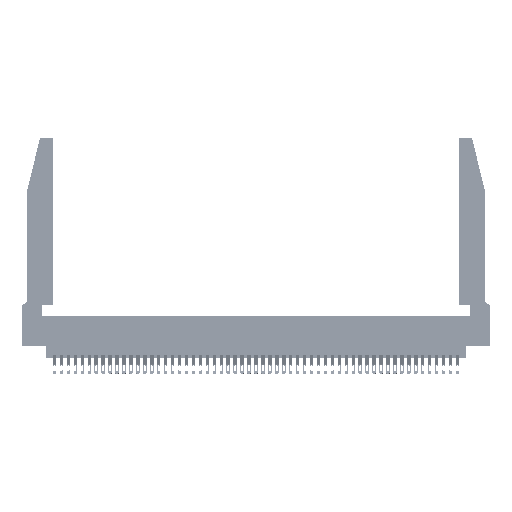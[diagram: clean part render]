
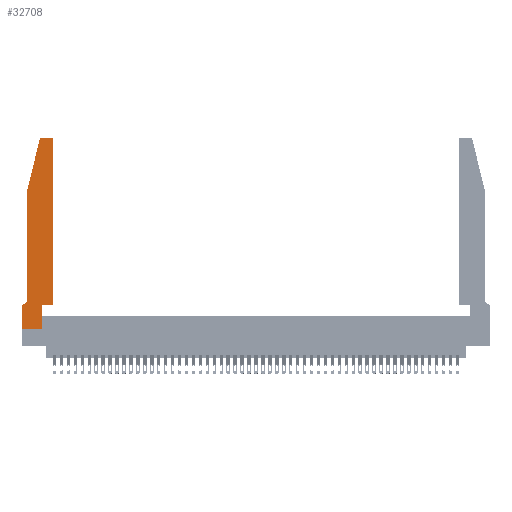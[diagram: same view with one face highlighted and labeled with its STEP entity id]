
A CAD part, top view. The second image highlights one B-rep face of the part: STEP entity #32708.
In plain terms, the highlighted planar face has unit normal (0, 0, 1).
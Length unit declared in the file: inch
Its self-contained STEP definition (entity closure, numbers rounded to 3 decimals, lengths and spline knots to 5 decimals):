
#137 = VERTEX_POINT ( 'NONE', #3479 ) ;
#506 = ORIENTED_EDGE ( 'NONE', *, *, #31045, .T. ) ;
#1207 = DIRECTION ( 'NONE',  ( 1., 0., 0. ) ) ;
#2155 = CARTESIAN_POINT ( 'NONE',  ( 0.0755, 2., 0.37 ) ) ;
#3479 = CARTESIAN_POINT ( 'NONE',  ( 0.2865, 0., 0.37 ) ) ;
#3508 = EDGE_CURVE ( 'NONE', #137, #24371, #4201, .T. ) ;
#4201 = LINE ( 'NONE', #27935, #20249 ) ;
#4368 = CARTESIAN_POINT ( 'NONE',  ( 0.0755, 2., 0.37 ) ) ;
#4693 = CARTESIAN_POINT ( 'NONE',  ( 0.0755, 0.42, 0.37 ) ) ;
#5701 = CARTESIAN_POINT ( 'NONE',  ( 0.0755, 2., 0.37 ) ) ;
#6188 = AXIS2_PLACEMENT_3D ( 'NONE', #13835, #40429, #44256 ) ;
#6487 = AXIS2_PLACEMENT_3D ( 'NONE', #41395, #21757, #26065 ) ;
#7069 = LINE ( 'NONE', #2155, #46385 ) ;
#8579 = CARTESIAN_POINT ( 'NONE',  ( 0.2865, 0.35, 0.37 ) ) ;
#10201 = CIRCLE ( 'NONE', #35204, 0.03 ) ;
#10376 = VECTOR ( 'NONE', #1207, 39.37008 ) ;
#10714 = CIRCLE ( 'NONE', #6188, 0.03 ) ;
#11457 = VERTEX_POINT ( 'NONE', #45460 ) ;
#11647 = LINE ( 'NONE', #43375, #15791 ) ;
#12059 = FACE_OUTER_BOUND ( 'NONE', #23910, .T. ) ;
#12420 = ORIENTED_EDGE ( 'NONE', *, *, #34769, .T. ) ;
#13361 = DIRECTION ( 'NONE',  ( 0., -1., 0. ) ) ;
#13835 = CARTESIAN_POINT ( 'NONE',  ( 0.4205, 2.72, 0.37 ) ) ;
#13990 = EDGE_CURVE ( 'NONE', #24371, #29983, #34779, .T. ) ;
#15791 = VECTOR ( 'NONE', #46891, 39.37008 ) ;
#15926 = VERTEX_POINT ( 'NONE', #24066 ) ;
#16414 = ORIENTED_EDGE ( 'NONE', *, *, #20562, .T. ) ;
#17161 = CARTESIAN_POINT ( 'NONE',  ( 0.4205, 2.75, 0.37 ) ) ;
#17663 = ORIENTED_EDGE ( 'NONE', *, *, #47077, .T. ) ;
#17779 = VERTEX_POINT ( 'NONE', #45844 ) ;
#18702 = CARTESIAN_POINT ( 'NONE',  ( 0.4505, 0.35, 0.37 ) ) ;
#19654 = VERTEX_POINT ( 'NONE', #4368 ) ;
#19939 = CARTESIAN_POINT ( 'NONE',  ( 0., 0., 0.37 ) ) ;
#20249 = VECTOR ( 'NONE', #40398, 39.37008 ) ;
#20545 = CARTESIAN_POINT ( 'NONE',  ( 0., 0., 0.37 ) ) ;
#20562 = EDGE_CURVE ( 'NONE', #17779, #137, #39783, .T. ) ;
#21757 = DIRECTION ( 'NONE',  ( 0., 0., -1. ) ) ;
#21945 = EDGE_CURVE ( 'NONE', #29983, #27282, #43775, .T. ) ;
#22101 = DIRECTION ( 'NONE',  ( 0., 0., 1. ) ) ;
#22217 = EDGE_CURVE ( 'NONE', #28894, #11457, #11647, .T. ) ;
#22573 = DIRECTION ( 'NONE',  ( 0., 1., 0. ) ) ;
#23110 = VECTOR ( 'NONE', #39688, 39.37008 ) ;
#23624 = CIRCLE ( 'NONE', #6487, 0.07 ) ;
#23910 = EDGE_LOOP ( 'NONE', ( #25880, #29594, #12420, #30678, #506, #31375, #17663, #16414, #26755, #45227, #28494, #25932 ) ) ;
#24066 = CARTESIAN_POINT ( 'NONE',  ( 0., 0.35, 0.37 ) ) ;
#24371 = VERTEX_POINT ( 'NONE', #8579 ) ;
#25573 = PLANE ( 'NONE',  #31054 ) ;
#25880 = ORIENTED_EDGE ( 'NONE', *, *, #22217, .T. ) ;
#25932 = ORIENTED_EDGE ( 'NONE', *, *, #29044, .T. ) ;
#26065 = DIRECTION ( 'NONE',  ( -1., 0., 0. ) ) ;
#26755 = ORIENTED_EDGE ( 'NONE', *, *, #3508, .T. ) ;
#27097 = VERTEX_POINT ( 'NONE', #4693 ) ;
#27282 = VERTEX_POINT ( 'NONE', #33248 ) ;
#27413 = CARTESIAN_POINT ( 'NONE',  ( 0.4505, 0.35, 0.37 ) ) ;
#27922 = LINE ( 'NONE', #5701, #40997 ) ;
#27935 = CARTESIAN_POINT ( 'NONE',  ( 0.2865, 0.35, 0.37 ) ) ;
#28453 = EDGE_CURVE ( 'NONE', #11457, #29487, #10201, .T. ) ;
#28494 = ORIENTED_EDGE ( 'NONE', *, *, #21945, .T. ) ;
#28683 = DIRECTION ( 'NONE',  ( -0.239, -0.971, 0. ) ) ;
#28894 = VERTEX_POINT ( 'NONE', #17161 ) ;
#28906 = CARTESIAN_POINT ( 'NONE',  ( 0.284, 2.72, 0.37 ) ) ;
#29044 = EDGE_CURVE ( 'NONE', #27282, #28894, #10714, .T. ) ;
#29487 = VERTEX_POINT ( 'NONE', #38893 ) ;
#29594 = ORIENTED_EDGE ( 'NONE', *, *, #28453, .T. ) ;
#29671 = VERTEX_POINT ( 'NONE', #39714 ) ;
#29983 = VERTEX_POINT ( 'NONE', #18702 ) ;
#30678 = ORIENTED_EDGE ( 'NONE', *, *, #34431, .T. ) ;
#31045 = EDGE_CURVE ( 'NONE', #27097, #29671, #23624, .T. ) ;
#31054 = AXIS2_PLACEMENT_3D ( 'NONE', #33600, #22101, #44415 ) ;
#31074 = VECTOR ( 'NONE', #42930, 39.37008 ) ;
#31375 = ORIENTED_EDGE ( 'NONE', *, *, #38452, .T. ) ;
#32708 = ADVANCED_FACE ( 'NONE', ( #12059 ), #25573, .T. ) ;
#33248 = CARTESIAN_POINT ( 'NONE',  ( 0.4505, 2.72, 0.37 ) ) ;
#33600 = CARTESIAN_POINT ( 'NONE',  ( 0., 0.35, 0.37 ) ) ;
#34431 = EDGE_CURVE ( 'NONE', #19654, #27097, #27922, .T. ) ;
#34582 = CARTESIAN_POINT ( 'NONE',  ( 0.0755, 0.35, 0.37 ) ) ;
#34769 = EDGE_CURVE ( 'NONE', #29487, #19654, #7069, .T. ) ;
#34779 = LINE ( 'NONE', #27413, #10376 ) ;
#35204 = AXIS2_PLACEMENT_3D ( 'NONE', #28906, #44389, #47580 ) ;
#37215 = VECTOR ( 'NONE', #22573, 39.37008 ) ;
#38452 = EDGE_CURVE ( 'NONE', #29671, #15926, #47821, .T. ) ;
#38893 = CARTESIAN_POINT ( 'NONE',  ( 0.25487, 2.72718, 0.37 ) ) ;
#39688 = DIRECTION ( 'NONE',  ( 1., 0., 0. ) ) ;
#39714 = CARTESIAN_POINT ( 'NONE',  ( 0.0055, 0.35, 0.37 ) ) ;
#39783 = LINE ( 'NONE', #20545, #23110 ) ;
#40398 = DIRECTION ( 'NONE',  ( 0., 1., 0. ) ) ;
#40429 = DIRECTION ( 'NONE',  ( 0., 0., 1. ) ) ;
#40596 = LINE ( 'NONE', #19939, #31074 ) ;
#40997 = VECTOR ( 'NONE', #13361, 39.37008 ) ;
#41395 = CARTESIAN_POINT ( 'NONE',  ( 0.0055, 0.42, 0.37 ) ) ;
#41727 = CARTESIAN_POINT ( 'NONE',  ( 0.4505, 0.35, 0.37 ) ) ;
#42930 = DIRECTION ( 'NONE',  ( 0., -1., 0. ) ) ;
#43375 = CARTESIAN_POINT ( 'NONE',  ( 0.2605, 2.75, 0.37 ) ) ;
#43775 = LINE ( 'NONE', #41727, #37215 ) ;
#44256 = DIRECTION ( 'NONE',  ( 1., 0., 0. ) ) ;
#44389 = DIRECTION ( 'NONE',  ( 0., 0., 1. ) ) ;
#44415 = DIRECTION ( 'NONE',  ( 1., 0., 0. ) ) ;
#45227 = ORIENTED_EDGE ( 'NONE', *, *, #13990, .T. ) ;
#45460 = CARTESIAN_POINT ( 'NONE',  ( 0.284, 2.75, 0.37 ) ) ;
#45844 = CARTESIAN_POINT ( 'NONE',  ( 0., 0., 0.37 ) ) ;
#46054 = DIRECTION ( 'NONE',  ( -1., 0., 0. ) ) ;
#46385 = VECTOR ( 'NONE', #28683, 39.37008 ) ;
#46891 = DIRECTION ( 'NONE',  ( -1., 0., 0. ) ) ;
#47077 = EDGE_CURVE ( 'NONE', #15926, #17779, #40596, .T. ) ;
#47251 = VECTOR ( 'NONE', #46054, 39.37008 ) ;
#47580 = DIRECTION ( 'NONE',  ( 1., 0., 0. ) ) ;
#47821 = LINE ( 'NONE', #34582, #47251 ) ;
